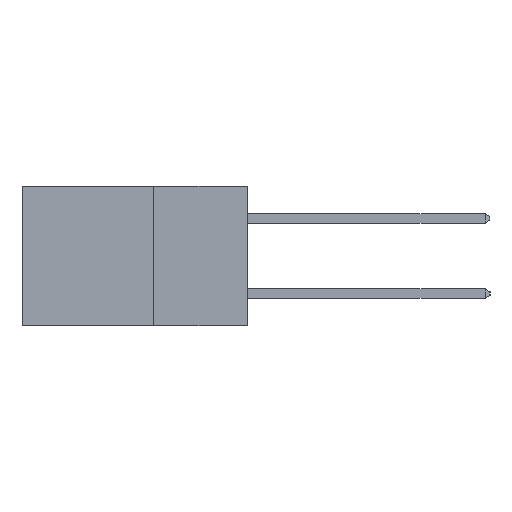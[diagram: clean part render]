
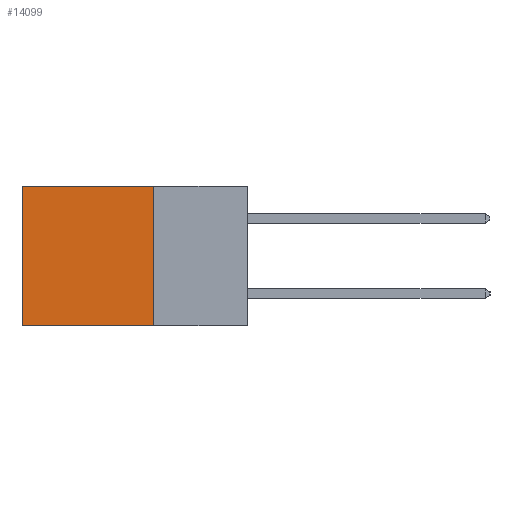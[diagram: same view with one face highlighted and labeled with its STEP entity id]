
A CAD part, left-side view. The second image highlights one B-rep face of the part: STEP entity #14099.
In plain terms, the highlighted planar face has unit normal (-1, 0, 0).
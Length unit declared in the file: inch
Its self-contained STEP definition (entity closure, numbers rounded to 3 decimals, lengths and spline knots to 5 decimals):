
#1206 = EDGE_CURVE ( 'NONE', #1349, #10987, #21266, .T. ) ;
#1349 = VERTEX_POINT ( 'NONE', #9103 ) ;
#3309 = LINE ( 'NONE', #9030, #7292 ) ;
#3592 = DIRECTION ( 'NONE',  ( 0., 0., -1. ) ) ;
#4343 = EDGE_CURVE ( 'NONE', #10987, #8853, #18083, .T. ) ;
#4853 = VECTOR ( 'NONE', #20498, 39.37008 ) ;
#5685 = VERTEX_POINT ( 'NONE', #21219 ) ;
#5929 = AXIS2_PLACEMENT_3D ( 'NONE', #18444, #8527, #20085 ) ;
#6884 = PLANE ( 'NONE',  #5929 ) ;
#7027 = ORIENTED_EDGE ( 'NONE', *, *, #14315, .T. ) ;
#7292 = VECTOR ( 'NONE', #17286, 39.37008 ) ;
#8527 = DIRECTION ( 'NONE',  ( 1., 0., 0. ) ) ;
#8561 = CARTESIAN_POINT ( 'NONE',  ( 0.2615, 0.6, -0.37 ) ) ;
#8853 = VERTEX_POINT ( 'NONE', #10130 ) ;
#9030 = CARTESIAN_POINT ( 'NONE',  ( 0.2615, 0.25, 0. ) ) ;
#9103 = CARTESIAN_POINT ( 'NONE',  ( 0.2615, 0.25, 0. ) ) ;
#10130 = CARTESIAN_POINT ( 'NONE',  ( 0.2615, 0.6, -0.37 ) ) ;
#10879 = EDGE_CURVE ( 'NONE', #5685, #8853, #16486, .T. ) ;
#10987 = VERTEX_POINT ( 'NONE', #12047 ) ;
#11695 = ORIENTED_EDGE ( 'NONE', *, *, #1206, .F. ) ;
#12047 = CARTESIAN_POINT ( 'NONE',  ( 0.2615, 0.25, -0.37 ) ) ;
#13034 = CARTESIAN_POINT ( 'NONE',  ( 0.2615, 0.25, -0.37 ) ) ;
#13215 = ORIENTED_EDGE ( 'NONE', *, *, #4343, .F. ) ;
#13259 = DIRECTION ( 'NONE',  ( 0., 0., -1. ) ) ;
#13666 = EDGE_LOOP ( 'NONE', ( #17290, #13215, #11695, #7027 ) ) ;
#14099 = ADVANCED_FACE ( 'NONE', ( #20204 ), #6884, .F. ) ;
#14315 = EDGE_CURVE ( 'NONE', #1349, #5685, #3309, .T. ) ;
#16416 = VECTOR ( 'NONE', #13259, 39.37008 ) ;
#16486 = LINE ( 'NONE', #8561, #20336 ) ;
#17286 = DIRECTION ( 'NONE',  ( 0., 1., 0. ) ) ;
#17290 = ORIENTED_EDGE ( 'NONE', *, *, #10879, .T. ) ;
#18083 = LINE ( 'NONE', #19603, #4853 ) ;
#18444 = CARTESIAN_POINT ( 'NONE',  ( 0.2615, 0.25, -0.37 ) ) ;
#19603 = CARTESIAN_POINT ( 'NONE',  ( 0.2615, 0.25, -0.37 ) ) ;
#20085 = DIRECTION ( 'NONE',  ( 0., 0., -1. ) ) ;
#20204 = FACE_OUTER_BOUND ( 'NONE', #13666, .T. ) ;
#20336 = VECTOR ( 'NONE', #3592, 39.37008 ) ;
#20498 = DIRECTION ( 'NONE',  ( 0., 1., 0. ) ) ;
#21219 = CARTESIAN_POINT ( 'NONE',  ( 0.2615, 0.6, 0. ) ) ;
#21266 = LINE ( 'NONE', #13034, #16416 ) ;
